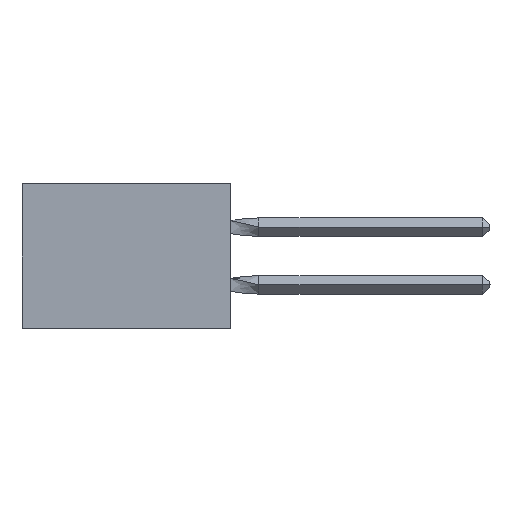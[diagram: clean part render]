
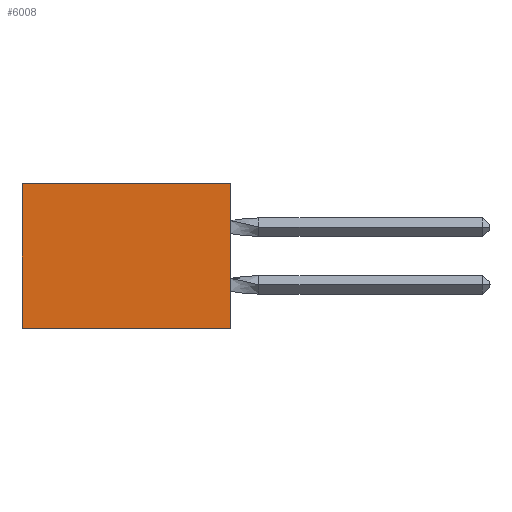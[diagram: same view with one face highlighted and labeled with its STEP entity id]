
A CAD part, left-side view. The second image highlights one B-rep face of the part: STEP entity #6008.
In plain terms, the highlighted planar face has unit normal (-1, 0, 0).
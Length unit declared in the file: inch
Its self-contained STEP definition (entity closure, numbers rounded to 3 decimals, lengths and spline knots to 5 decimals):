
#163 = DIRECTION ( 'NONE',  ( 1., 0., 0. ) ) ;
#571 = LINE ( 'NONE', #7623, #17340 ) ;
#671 = DIRECTION ( 'NONE',  ( 0., 1., 0. ) ) ;
#1928 = EDGE_CURVE ( 'NONE', #18501, #9132, #3801, .T. ) ;
#2231 = CARTESIAN_POINT ( 'NONE',  ( 0.305, 0., 0. ) ) ;
#3000 = ORIENTED_EDGE ( 'NONE', *, *, #17143, .T. ) ;
#3267 = LINE ( 'NONE', #3622, #13327 ) ;
#3484 = DIRECTION ( 'NONE',  ( 0., 1., 0. ) ) ;
#3622 = CARTESIAN_POINT ( 'NONE',  ( 0.305, 0.72, -0.5 ) ) ;
#3801 = LINE ( 'NONE', #15582, #14972 ) ;
#5046 = DIRECTION ( 'NONE',  ( 0., 0., -1. ) ) ;
#5328 = CARTESIAN_POINT ( 'NONE',  ( 0.305, 0.72, -0.5 ) ) ;
#6008 = ADVANCED_FACE ( 'NONE', ( #14184 ), #8745, .F. ) ;
#6170 = VERTEX_POINT ( 'NONE', #9286 ) ;
#7623 = CARTESIAN_POINT ( 'NONE',  ( 0.305, 0., -0.5 ) ) ;
#7995 = VERTEX_POINT ( 'NONE', #5328 ) ;
#8685 = ORIENTED_EDGE ( 'NONE', *, *, #13812, .T. ) ;
#8745 = PLANE ( 'NONE',  #9130 ) ;
#9130 = AXIS2_PLACEMENT_3D ( 'NONE', #11711, #163, #13228 ) ;
#9132 = VERTEX_POINT ( 'NONE', #15565 ) ;
#9286 = CARTESIAN_POINT ( 'NONE',  ( 0.305, 0.72, 0. ) ) ;
#10475 = LINE ( 'NONE', #2231, #12474 ) ;
#11711 = CARTESIAN_POINT ( 'NONE',  ( 0.305, 0., -0.5 ) ) ;
#12474 = VECTOR ( 'NONE', #671, 39.37008 ) ;
#13228 = DIRECTION ( 'NONE',  ( 0., 0., -1. ) ) ;
#13234 = EDGE_LOOP ( 'NONE', ( #8685, #17147, #14133, #3000 ) ) ;
#13327 = VECTOR ( 'NONE', #5046, 39.37008 ) ;
#13812 = EDGE_CURVE ( 'NONE', #6170, #7995, #3267, .T. ) ;
#14133 = ORIENTED_EDGE ( 'NONE', *, *, #1928, .F. ) ;
#14184 = FACE_OUTER_BOUND ( 'NONE', #13234, .T. ) ;
#14335 = EDGE_CURVE ( 'NONE', #9132, #7995, #571, .T. ) ;
#14972 = VECTOR ( 'NONE', #18393, 39.37008 ) ;
#15357 = CARTESIAN_POINT ( 'NONE',  ( 0.305, 0., 0. ) ) ;
#15565 = CARTESIAN_POINT ( 'NONE',  ( 0.305, 0., -0.5 ) ) ;
#15582 = CARTESIAN_POINT ( 'NONE',  ( 0.305, 0., -0.5 ) ) ;
#17143 = EDGE_CURVE ( 'NONE', #18501, #6170, #10475, .T. ) ;
#17147 = ORIENTED_EDGE ( 'NONE', *, *, #14335, .F. ) ;
#17340 = VECTOR ( 'NONE', #3484, 39.37008 ) ;
#18393 = DIRECTION ( 'NONE',  ( 0., 0., -1. ) ) ;
#18501 = VERTEX_POINT ( 'NONE', #15357 ) ;
